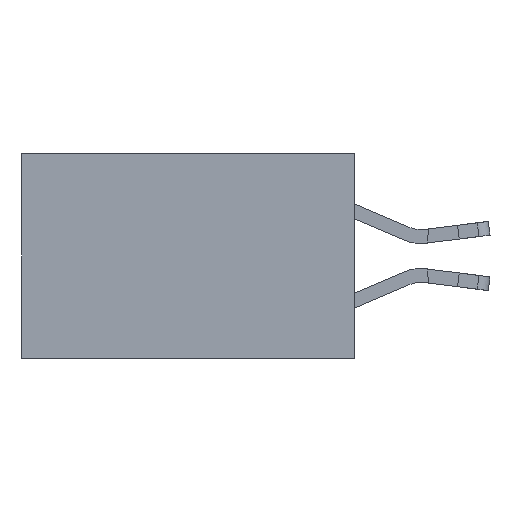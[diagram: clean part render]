
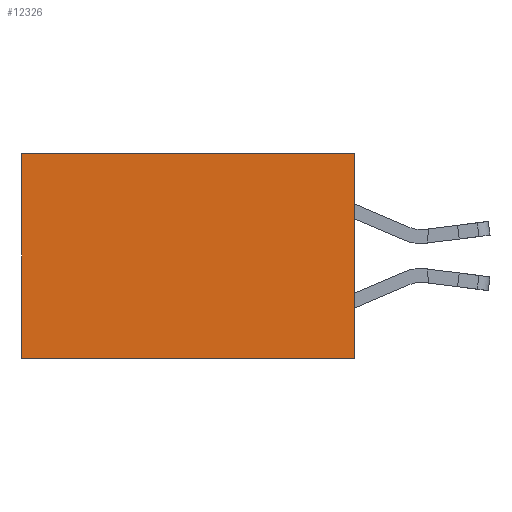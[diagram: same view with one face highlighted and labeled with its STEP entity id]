
A CAD part, left-side view. The second image highlights one B-rep face of the part: STEP entity #12326.
In plain terms, the highlighted planar face has unit normal (-1, 0, 0).
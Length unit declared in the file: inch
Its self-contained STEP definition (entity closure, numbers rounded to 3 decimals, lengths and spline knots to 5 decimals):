
#176 = LINE ( 'NONE', #10921, #13512 ) ;
#2834 = LINE ( 'NONE', #9371, #21153 ) ;
#3550 = CARTESIAN_POINT ( 'NONE',  ( 0.298, 0.6, 0. ) ) ;
#4091 = DIRECTION ( 'NONE',  ( 0., 1., 0. ) ) ;
#4101 = ORIENTED_EDGE ( 'NONE', *, *, #17607, .T. ) ;
#4585 = CARTESIAN_POINT ( 'NONE',  ( 0.298, 0., 0. ) ) ;
#5424 = ORIENTED_EDGE ( 'NONE', *, *, #12037, .F. ) ;
#5785 = VERTEX_POINT ( 'NONE', #13461 ) ;
#5923 = VECTOR ( 'NONE', #10749, 39.37008 ) ;
#6617 = VERTEX_POINT ( 'NONE', #3550 ) ;
#7237 = CARTESIAN_POINT ( 'NONE',  ( 0.298, 0.6, 0. ) ) ;
#7374 = VERTEX_POINT ( 'NONE', #12502 ) ;
#7475 = DIRECTION ( 'NONE',  ( 0., 1., 0. ) ) ;
#8455 = LINE ( 'NONE', #4585, #17633 ) ;
#8525 = PLANE ( 'NONE',  #11713 ) ;
#8591 = VERTEX_POINT ( 'NONE', #10722 ) ;
#9371 = CARTESIAN_POINT ( 'NONE',  ( 0.298, 0., 0. ) ) ;
#10304 = DIRECTION ( 'NONE',  ( 1., 0., 0. ) ) ;
#10573 = LINE ( 'NONE', #7237, #5923 ) ;
#10722 = CARTESIAN_POINT ( 'NONE',  ( 0.298, 0., -0.37 ) ) ;
#10749 = DIRECTION ( 'NONE',  ( 0., 0., -1. ) ) ;
#10921 = CARTESIAN_POINT ( 'NONE',  ( 0.298, 0., -0.37 ) ) ;
#11002 = ORIENTED_EDGE ( 'NONE', *, *, #15898, .T. ) ;
#11713 = AXIS2_PLACEMENT_3D ( 'NONE', #18836, #10304, #22183 ) ;
#12037 = EDGE_CURVE ( 'NONE', #8591, #7374, #176, .T. ) ;
#12326 = ADVANCED_FACE ( 'NONE', ( #16732 ), #8525, .F. ) ;
#12499 = ORIENTED_EDGE ( 'NONE', *, *, #13589, .F. ) ;
#12502 = CARTESIAN_POINT ( 'NONE',  ( 0.298, 0.6, -0.37 ) ) ;
#13461 = CARTESIAN_POINT ( 'NONE',  ( 0.298, 0., 0. ) ) ;
#13512 = VECTOR ( 'NONE', #7475, 39.37008 ) ;
#13589 = EDGE_CURVE ( 'NONE', #5785, #8591, #8455, .T. ) ;
#14976 = DIRECTION ( 'NONE',  ( 0., 0., -1. ) ) ;
#15898 = EDGE_CURVE ( 'NONE', #6617, #7374, #10573, .T. ) ;
#16732 = FACE_OUTER_BOUND ( 'NONE', #21827, .T. ) ;
#17607 = EDGE_CURVE ( 'NONE', #5785, #6617, #2834, .T. ) ;
#17633 = VECTOR ( 'NONE', #14976, 39.37008 ) ;
#18836 = CARTESIAN_POINT ( 'NONE',  ( 0.298, 0., 0. ) ) ;
#21153 = VECTOR ( 'NONE', #4091, 39.37008 ) ;
#21827 = EDGE_LOOP ( 'NONE', ( #11002, #5424, #12499, #4101 ) ) ;
#22183 = DIRECTION ( 'NONE',  ( 0., 0., -1. ) ) ;
